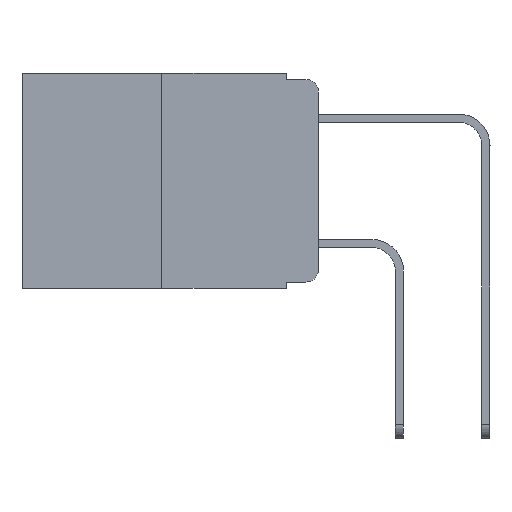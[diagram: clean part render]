
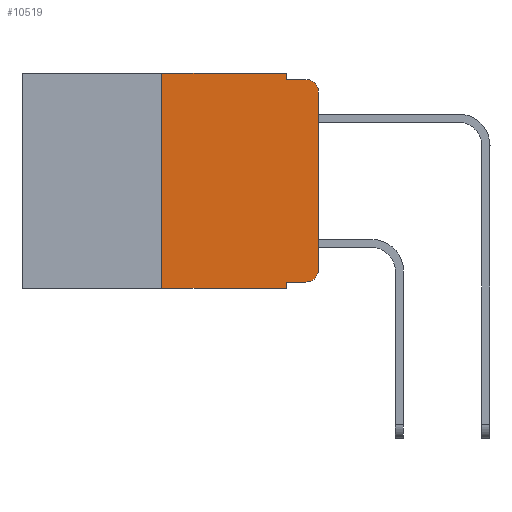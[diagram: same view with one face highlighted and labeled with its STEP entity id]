
A CAD part, left-side view. The second image highlights one B-rep face of the part: STEP entity #10519.
In plain terms, the highlighted planar face has unit normal (-1, 0, 0).
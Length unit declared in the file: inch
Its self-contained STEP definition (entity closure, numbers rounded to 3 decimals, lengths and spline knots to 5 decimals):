
#530 = DIRECTION ( 'NONE',  ( 0., 0., -1. ) ) ;
#577 = VERTEX_POINT ( 'NONE', #1467 ) ;
#724 = EDGE_CURVE ( 'NONE', #6732, #11465, #11326, .T. ) ;
#937 = EDGE_CURVE ( 'NONE', #14795, #11465, #5066, .T. ) ;
#1431 = ORIENTED_EDGE ( 'NONE', *, *, #12244, .T. ) ;
#1467 = CARTESIAN_POINT ( 'NONE',  ( 0., 0., -0.313 ) ) ;
#1491 = VECTOR ( 'NONE', #12881, 39.37008 ) ;
#1687 = CARTESIAN_POINT ( 'NONE',  ( 0., 0.25, 0. ) ) ;
#1700 = EDGE_CURVE ( 'NONE', #14795, #13702, #6231, .T. ) ;
#1859 = LINE ( 'NONE', #11433, #19073 ) ;
#2340 = DIRECTION ( 'NONE',  ( 0., -1., 0. ) ) ;
#2341 = DIRECTION ( 'NONE',  ( 1., 0., 0. ) ) ;
#2572 = EDGE_CURVE ( 'NONE', #6732, #14879, #12354, .T. ) ;
#3089 = VECTOR ( 'NONE', #7763, 39.37008 ) ;
#3541 = CARTESIAN_POINT ( 'NONE',  ( 0., 0.051, 0. ) ) ;
#3847 = CARTESIAN_POINT ( 'NONE',  ( 0., 0.02, -0.01 ) ) ;
#4443 = CARTESIAN_POINT ( 'NONE',  ( 0., 0.02, -0.333 ) ) ;
#4571 = CIRCLE ( 'NONE', #18036, 0.02 ) ;
#4578 = VECTOR ( 'NONE', #19372, 39.37008 ) ;
#5066 = LINE ( 'NONE', #7074, #11801 ) ;
#5327 = ORIENTED_EDGE ( 'NONE', *, *, #724, .F. ) ;
#5411 = CARTESIAN_POINT ( 'NONE',  ( 0., 0.051, -0.333 ) ) ;
#5701 = EDGE_CURVE ( 'NONE', #9411, #11845, #18301, .T. ) ;
#6132 = CARTESIAN_POINT ( 'NONE',  ( 0., 0.25, 0. ) ) ;
#6231 = LINE ( 'NONE', #6132, #3089 ) ;
#6501 = VECTOR ( 'NONE', #20086, 39.37008 ) ;
#6619 = VECTOR ( 'NONE', #17094, 39.37008 ) ;
#6732 = VERTEX_POINT ( 'NONE', #5411 ) ;
#6777 = VECTOR ( 'NONE', #530, 39.37008 ) ;
#7074 = CARTESIAN_POINT ( 'NONE',  ( 0., 0.473, -0.343 ) ) ;
#7121 = EDGE_CURVE ( 'NONE', #13702, #8006, #8330, .T. ) ;
#7697 = CARTESIAN_POINT ( 'NONE',  ( 0., 0.051, -0.01 ) ) ;
#7763 = DIRECTION ( 'NONE',  ( 0., 0., 1. ) ) ;
#8006 = VERTEX_POINT ( 'NONE', #17856 ) ;
#8330 = LINE ( 'NONE', #12526, #6619 ) ;
#8684 = LINE ( 'NONE', #19577, #4578 ) ;
#9018 = DIRECTION ( 'NONE',  ( 0., 0., -1. ) ) ;
#9411 = VERTEX_POINT ( 'NONE', #18055 ) ;
#9523 = EDGE_LOOP ( 'NONE', ( #11767, #15193, #10030, #14149, #17235, #12322, #13465, #5327, #10748, #1431 ) ) ;
#9929 = CARTESIAN_POINT ( 'NONE',  ( 0., 0.051, -0.333 ) ) ;
#10030 = ORIENTED_EDGE ( 'NONE', *, *, #18100, .F. ) ;
#10232 = VERTEX_POINT ( 'NONE', #7697 ) ;
#10519 = ADVANCED_FACE ( 'NONE', ( #13807 ), #13195, .F. ) ;
#10748 = ORIENTED_EDGE ( 'NONE', *, *, #2572, .T. ) ;
#11326 = LINE ( 'NONE', #13828, #6501 ) ;
#11433 = CARTESIAN_POINT ( 'NONE',  ( 0., 0., 0. ) ) ;
#11465 = VERTEX_POINT ( 'NONE', #13619 ) ;
#11767 = ORIENTED_EDGE ( 'NONE', *, *, #12602, .T. ) ;
#11801 = VECTOR ( 'NONE', #2340, 39.37008 ) ;
#11845 = VERTEX_POINT ( 'NONE', #3847 ) ;
#12244 = EDGE_CURVE ( 'NONE', #14879, #577, #4571, .T. ) ;
#12322 = ORIENTED_EDGE ( 'NONE', *, *, #1700, .F. ) ;
#12354 = LINE ( 'NONE', #9929, #1491 ) ;
#12526 = CARTESIAN_POINT ( 'NONE',  ( 0., 0.473, 0. ) ) ;
#12602 = EDGE_CURVE ( 'NONE', #577, #9411, #1859, .T. ) ;
#12881 = DIRECTION ( 'NONE',  ( 0., -1., 0. ) ) ;
#13195 = PLANE ( 'NONE',  #16312 ) ;
#13465 = ORIENTED_EDGE ( 'NONE', *, *, #937, .T. ) ;
#13619 = CARTESIAN_POINT ( 'NONE',  ( 0., 0.051, -0.343 ) ) ;
#13702 = VERTEX_POINT ( 'NONE', #1687 ) ;
#13807 = FACE_OUTER_BOUND ( 'NONE', #9523, .T. ) ;
#13828 = CARTESIAN_POINT ( 'NONE',  ( 0., 0.051, 0. ) ) ;
#14149 = ORIENTED_EDGE ( 'NONE', *, *, #16044, .F. ) ;
#14602 = DIRECTION ( 'NONE',  ( -1., 0., 0. ) ) ;
#14795 = VERTEX_POINT ( 'NONE', #15382 ) ;
#14879 = VERTEX_POINT ( 'NONE', #4443 ) ;
#15193 = ORIENTED_EDGE ( 'NONE', *, *, #5701, .T. ) ;
#15367 = DIRECTION ( 'NONE',  ( -1., 0., 0. ) ) ;
#15382 = CARTESIAN_POINT ( 'NONE',  ( 0., 0.25, -0.343 ) ) ;
#16044 = EDGE_CURVE ( 'NONE', #8006, #10232, #18414, .T. ) ;
#16170 = DIRECTION ( 'NONE',  ( 0., 0., -1. ) ) ;
#16312 = AXIS2_PLACEMENT_3D ( 'NONE', #19538, #2341, #17826 ) ;
#16798 = CARTESIAN_POINT ( 'NONE',  ( 0., 0.02, -0.03 ) ) ;
#17094 = DIRECTION ( 'NONE',  ( 0., -1., 0. ) ) ;
#17235 = ORIENTED_EDGE ( 'NONE', *, *, #7121, .F. ) ;
#17671 = AXIS2_PLACEMENT_3D ( 'NONE', #16798, #15367, #9018 ) ;
#17826 = DIRECTION ( 'NONE',  ( 0., 0., -1. ) ) ;
#17856 = CARTESIAN_POINT ( 'NONE',  ( 0., 0.051, 0. ) ) ;
#18036 = AXIS2_PLACEMENT_3D ( 'NONE', #19306, #14602, #16170 ) ;
#18055 = CARTESIAN_POINT ( 'NONE',  ( 0., 0., -0.03 ) ) ;
#18100 = EDGE_CURVE ( 'NONE', #10232, #11845, #8684, .T. ) ;
#18301 = CIRCLE ( 'NONE', #17671, 0.02 ) ;
#18414 = LINE ( 'NONE', #3541, #6777 ) ;
#19073 = VECTOR ( 'NONE', #19440, 39.37008 ) ;
#19306 = CARTESIAN_POINT ( 'NONE',  ( 0., 0.02, -0.313 ) ) ;
#19372 = DIRECTION ( 'NONE',  ( 0., -1., 0. ) ) ;
#19440 = DIRECTION ( 'NONE',  ( 0., 0., 1. ) ) ;
#19538 = CARTESIAN_POINT ( 'NONE',  ( 0., 0.473, 0. ) ) ;
#19577 = CARTESIAN_POINT ( 'NONE',  ( 0., 0.051, -0.01 ) ) ;
#20086 = DIRECTION ( 'NONE',  ( 0., 0., -1. ) ) ;
